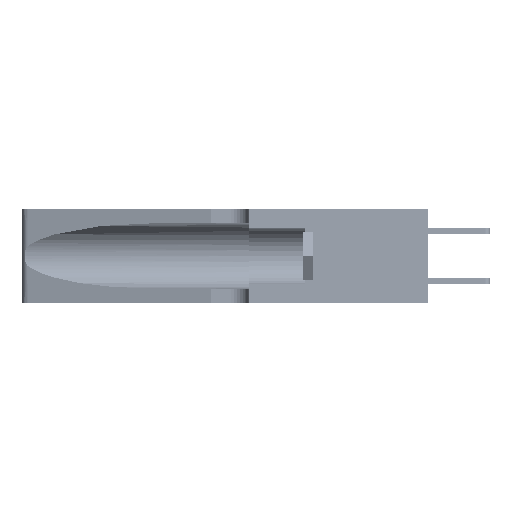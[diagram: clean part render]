
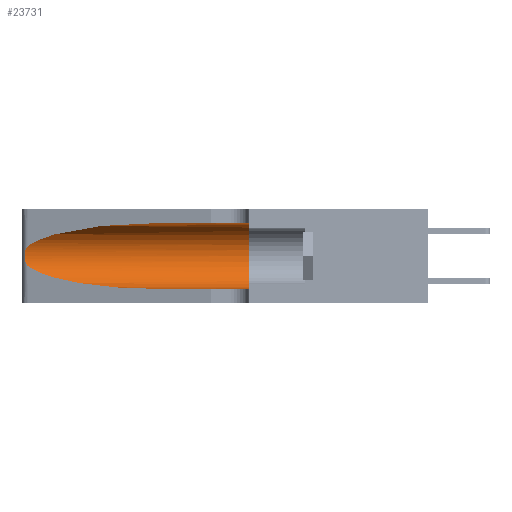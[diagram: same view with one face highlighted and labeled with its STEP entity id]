
A CAD part, left-side view. The second image highlights one B-rep face of the part: STEP entity #23731.
In plain terms, the highlighted cylindrical face has radius 3.308 mm (diameter 6.617 mm), a partial arc.
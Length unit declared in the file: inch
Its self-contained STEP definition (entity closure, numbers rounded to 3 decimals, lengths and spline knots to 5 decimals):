
#40 = ORIENTED_EDGE ( 'NONE', *, *, #18831, .T. ) ;
#678 = LINE ( 'NONE', #12478, #18661 ) ;
#695 = FACE_OUTER_BOUND ( 'NONE', #36523, .T. ) ;
#928 = CARTESIAN_POINT ( 'NONE',  ( 0.1305, 1.61858, 0.185 ) ) ;
#1407 = CARTESIAN_POINT ( 'NONE',  ( 0.1305, 0.35, 0.05475 ) ) ;
#1622 = CARTESIAN_POINT ( 'NONE',  ( 0.25555, 1.22993, 0.14849 ) ) ;
#2769 = CARTESIAN_POINT ( 'NONE',  ( 0.1305, 0.72297, 0.05475 ) ) ;
#3853 = ORIENTED_EDGE ( 'NONE', *, *, #7672, .T. ) ;
#4075 = ORIENTED_EDGE ( 'NONE', *, *, #40509, .T. ) ;
#4576 = CARTESIAN_POINT ( 'NONE',  ( 0.25487, 1.22718, 0.22369 ) ) ;
#4637 = CARTESIAN_POINT ( 'NONE',  ( 0.25487, 1.22718, 0.14631 ) ) ;
#4642 = CARTESIAN_POINT ( 'NONE',  ( 0.18966, 0.96281, 0.31525 ) ) ;
#4865 = CARTESIAN_POINT ( 'NONE',  ( 0.26075, 1.23896, 0.19203 ) ) ;
#5478 = VERTEX_POINT ( 'NONE', #13800 ) ;
#7672 = EDGE_CURVE ( 'NONE', #32174, #10853, #8253, .T. ) ;
#7986 = CARTESIAN_POINT ( 'NONE',  ( 0.25555, 1.22994, 0.2215 ) ) ;
#8253 =( BOUNDED_CURVE ( )  B_SPLINE_CURVE ( 3, ( #4637, #27681, #14269, #37799 ),
 .UNSPECIFIED., .F., .F. ) 
 B_SPLINE_CURVE_WITH_KNOTS ( ( 4, 4 ),
 ( 3.44316, 4.71239 ),
 .UNSPECIFIED. ) 
 CURVE ( )  GEOMETRIC_REPRESENTATION_ITEM ( )  RATIONAL_B_SPLINE_CURVE ( ( 1., 0.87, 0.87, 1. ) ) 
 REPRESENTATION_ITEM ( '' )  );
#8450 = CARTESIAN_POINT ( 'NONE',  ( 0.1305, 0.35, 0.185 ) ) ;
#8866 = CARTESIAN_POINT ( 'NONE',  ( 0.25639, 1.23186, 0.15144 ) ) ;
#10152 =( BOUNDED_CURVE ( )  B_SPLINE_CURVE ( 3, ( #21484, #4642, #41063, #14272 ),
 .UNSPECIFIED., .F., .T. ) 
 B_SPLINE_CURVE_WITH_KNOTS ( ( 4, 4 ),
 ( 1.5708, 2.84003 ),
 .UNSPECIFIED. ) 
 CURVE ( )  GEOMETRIC_REPRESENTATION_ITEM ( )  RATIONAL_B_SPLINE_CURVE ( ( 1., 0.87, 0.87, 1. ) ) 
 REPRESENTATION_ITEM ( '' )  );
#10853 = VERTEX_POINT ( 'NONE', #2769 ) ;
#11875 = DIRECTION ( 'NONE',  ( 0., 0., 1. ) ) ;
#11983 = CARTESIAN_POINT ( 'NONE',  ( 0.25789, 1.23486, 0.15765 ) ) ;
#12478 = CARTESIAN_POINT ( 'NONE',  ( 0.1305, 1.61858, 0.05475 ) ) ;
#12934 = CARTESIAN_POINT ( 'NONE',  ( 0.25487, 1.22718, 0.22369 ) ) ;
#13800 = CARTESIAN_POINT ( 'NONE',  ( 0.1305, 0.72297, 0.31525 ) ) ;
#13922 = CYLINDRICAL_SURFACE ( 'NONE', #32588, 0.13025 ) ;
#14223 = DIRECTION ( 'NONE',  ( 0., 0., -1. ) ) ;
#14269 = CARTESIAN_POINT ( 'NONE',  ( 0.18966, 0.96281, 0.05475 ) ) ;
#14272 = CARTESIAN_POINT ( 'NONE',  ( 0.25487, 1.22718, 0.22369 ) ) ;
#14450 = LINE ( 'NONE', #20685, #38095 ) ;
#14522 = CARTESIAN_POINT ( 'NONE',  ( 0.25856, 1.23593, 0.16098 ) ) ;
#17871 = CARTESIAN_POINT ( 'NONE',  ( 0.1305, 0.35, 0.31525 ) ) ;
#18561 = B_SPLINE_CURVE_WITH_KNOTS ( 'NONE', 3,
 ( #4576, #7986, #41742, #24955, #25111, #35128, #4865, #35248, #31306, #14522, #11983, #8866, #1622, #22128 ),
 .UNSPECIFIED., .F., .F.,
 ( 4, 2, 2, 2, 2, 2, 4 ),
 ( 0., 0.00027, 0.00053, 0.00107, 0.0016, 0.00187, 0.00214 ),
 .UNSPECIFIED. ) ;
#18661 = VECTOR ( 'NONE', #26301, 39.37008 ) ;
#18831 = EDGE_CURVE ( 'NONE', #5478, #33939, #10152, .T. ) ;
#19491 = AXIS2_PLACEMENT_3D ( 'NONE', #8450, #28512, #11875 ) ;
#20067 = VERTEX_POINT ( 'NONE', #17871 ) ;
#20685 = CARTESIAN_POINT ( 'NONE',  ( 0.1305, 1.61858, 0.31525 ) ) ;
#20842 = DIRECTION ( 'NONE',  ( 0., -1., 0. ) ) ;
#21484 = CARTESIAN_POINT ( 'NONE',  ( 0.1305, 0.72297, 0.31525 ) ) ;
#21686 = EDGE_CURVE ( 'NONE', #5478, #20067, #14450, .T. ) ;
#22128 = CARTESIAN_POINT ( 'NONE',  ( 0.25487, 1.22718, 0.14631 ) ) ;
#23465 = CIRCLE ( 'NONE', #19491, 0.13025 ) ;
#23731 = ADVANCED_FACE ( 'NONE', ( #695 ), #13922, .F. ) ;
#24955 = CARTESIAN_POINT ( 'NONE',  ( 0.25787, 1.23484, 0.2124 ) ) ;
#25111 = CARTESIAN_POINT ( 'NONE',  ( 0.25854, 1.2359, 0.20912 ) ) ;
#26301 = DIRECTION ( 'NONE',  ( 0., -1., 0. ) ) ;
#27681 = CARTESIAN_POINT ( 'NONE',  ( 0.2373, 1.15595, 0.08982 ) ) ;
#27834 = CARTESIAN_POINT ( 'NONE',  ( 0.25487, 1.22718, 0.14631 ) ) ;
#27875 = ORIENTED_EDGE ( 'NONE', *, *, #28469, .T. ) ;
#28469 = EDGE_CURVE ( 'NONE', #33939, #32174, #18561, .T. ) ;
#28512 = DIRECTION ( 'NONE',  ( 0., 1., 0. ) ) ;
#31054 = EDGE_CURVE ( 'NONE', #20067, #40365, #23465, .T. ) ;
#31306 = CARTESIAN_POINT ( 'NONE',  ( 0.26017, 1.23833, 0.17102 ) ) ;
#31330 = DIRECTION ( 'NONE',  ( 0., -1., 0. ) ) ;
#32174 = VERTEX_POINT ( 'NONE', #27834 ) ;
#32588 = AXIS2_PLACEMENT_3D ( 'NONE', #928, #31330, #14223 ) ;
#33939 = VERTEX_POINT ( 'NONE', #12934 ) ;
#35128 = CARTESIAN_POINT ( 'NONE',  ( 0.26018, 1.23835, 0.19895 ) ) ;
#35248 = CARTESIAN_POINT ( 'NONE',  ( 0.26075, 1.23896, 0.178 ) ) ;
#36523 = EDGE_LOOP ( 'NONE', ( #40, #27875, #3853, #4075, #41507, #39302 ) ) ;
#37799 = CARTESIAN_POINT ( 'NONE',  ( 0.1305, 0.72297, 0.05475 ) ) ;
#38095 = VECTOR ( 'NONE', #20842, 39.37008 ) ;
#39302 = ORIENTED_EDGE ( 'NONE', *, *, #21686, .F. ) ;
#40365 = VERTEX_POINT ( 'NONE', #1407 ) ;
#40509 = EDGE_CURVE ( 'NONE', #10853, #40365, #678, .T. ) ;
#41063 = CARTESIAN_POINT ( 'NONE',  ( 0.2373, 1.15595, 0.28018 ) ) ;
#41507 = ORIENTED_EDGE ( 'NONE', *, *, #31054, .F. ) ;
#41742 = CARTESIAN_POINT ( 'NONE',  ( 0.25639, 1.23184, 0.21858 ) ) ;
